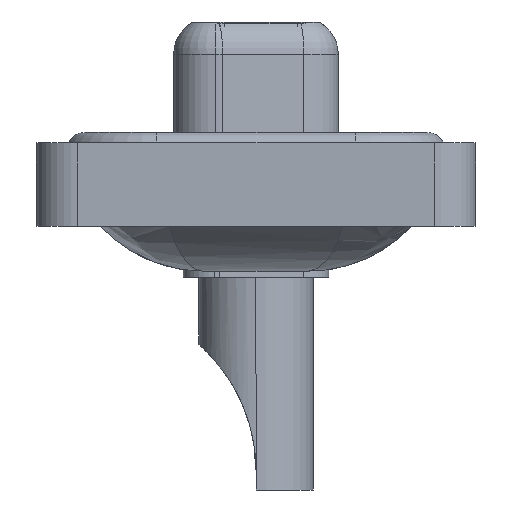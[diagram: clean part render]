
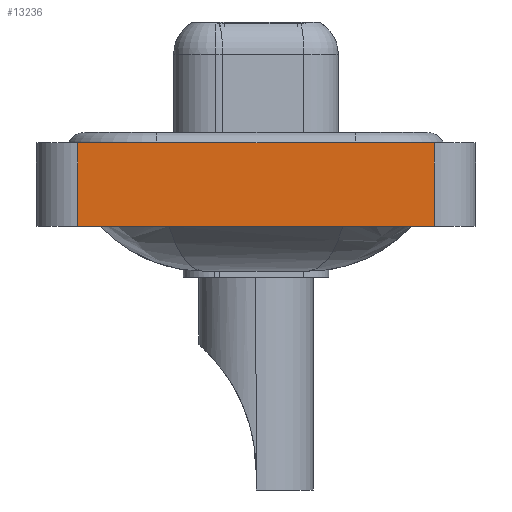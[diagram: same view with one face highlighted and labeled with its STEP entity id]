
A CAD part, left-side view. The second image highlights one B-rep face of the part: STEP entity #13236.
In plain terms, the highlighted planar face has unit normal (-1, 0, 0).
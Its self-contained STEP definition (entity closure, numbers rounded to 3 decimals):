
#1619 = LINE ( 'NONE', #15569, #20045 ) ;
#1733 = DIRECTION ( 'NONE',  ( 0., 0., 1. ) ) ;
#2146 = CARTESIAN_POINT ( 'NONE',  ( -7.35, 8.55, 0.4 ) ) ;
#2491 = CARTESIAN_POINT ( 'NONE',  ( -7.35, -8.55, -3.6 ) ) ;
#2558 = DIRECTION ( 'NONE',  ( 0., -1., 0. ) ) ;
#3798 = VECTOR ( 'NONE', #8879, 1000. ) ;
#4220 = EDGE_CURVE ( 'NONE', #17033, #14579, #7153, .T. ) ;
#5754 = CARTESIAN_POINT ( 'NONE',  ( -7.35, -8.55, -3.6 ) ) ;
#6642 = AXIS2_PLACEMENT_3D ( 'NONE', #2491, #9961, #8120 ) ;
#7153 = LINE ( 'NONE', #9002, #3798 ) ;
#7595 = LINE ( 'NONE', #5754, #16701 ) ;
#8120 = DIRECTION ( 'NONE',  ( 0., 0., 1. ) ) ;
#8812 = EDGE_CURVE ( 'NONE', #14579, #14624, #7595, .T. ) ;
#8879 = DIRECTION ( 'NONE',  ( 0., -1., 0. ) ) ;
#9002 = CARTESIAN_POINT ( 'NONE',  ( -7.35, -8.55, -3.6 ) ) ;
#9255 = ORIENTED_EDGE ( 'NONE', *, *, #4220, .T. ) ;
#9445 = DIRECTION ( 'NONE',  ( 0., 0., 1. ) ) ;
#9672 = EDGE_LOOP ( 'NONE', ( #13996, #12345, #19837, #9255 ) ) ;
#9961 = DIRECTION ( 'NONE',  ( -1., 0., 0. ) ) ;
#11477 = CARTESIAN_POINT ( 'NONE',  ( -7.35, -8.55, 0.4 ) ) ;
#11598 = FACE_OUTER_BOUND ( 'NONE', #9672, .T. ) ;
#11819 = CARTESIAN_POINT ( 'NONE',  ( -7.35, -8.55, -3.6 ) ) ;
#12345 = ORIENTED_EDGE ( 'NONE', *, *, #16605, .F. ) ;
#13236 = ADVANCED_FACE ( 'NONE', ( #11598 ), #18380, .T. ) ;
#13277 = CARTESIAN_POINT ( 'NONE',  ( -7.35, -8.55, 0.4 ) ) ;
#13400 = LINE ( 'NONE', #13277, #14898 ) ;
#13996 = ORIENTED_EDGE ( 'NONE', *, *, #8812, .T. ) ;
#14579 = VERTEX_POINT ( 'NONE', #11819 ) ;
#14624 = VERTEX_POINT ( 'NONE', #11477 ) ;
#14898 = VECTOR ( 'NONE', #2558, 1000. ) ;
#15569 = CARTESIAN_POINT ( 'NONE',  ( -7.35, 8.55, -3.6 ) ) ;
#16605 = EDGE_CURVE ( 'NONE', #18035, #14624, #13400, .T. ) ;
#16701 = VECTOR ( 'NONE', #9445, 1000. ) ;
#17033 = VERTEX_POINT ( 'NONE', #17198 ) ;
#17198 = CARTESIAN_POINT ( 'NONE',  ( -7.35, 8.55, -3.6 ) ) ;
#17318 = EDGE_CURVE ( 'NONE', #17033, #18035, #1619, .T. ) ;
#18035 = VERTEX_POINT ( 'NONE', #2146 ) ;
#18380 = PLANE ( 'NONE',  #6642 ) ;
#19837 = ORIENTED_EDGE ( 'NONE', *, *, #17318, .F. ) ;
#20045 = VECTOR ( 'NONE', #1733, 1000. ) ;
